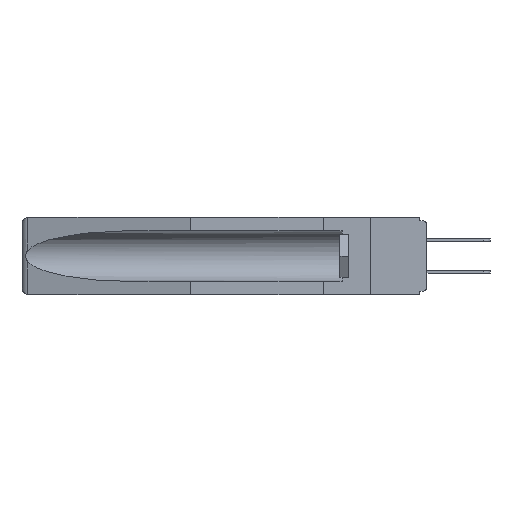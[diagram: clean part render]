
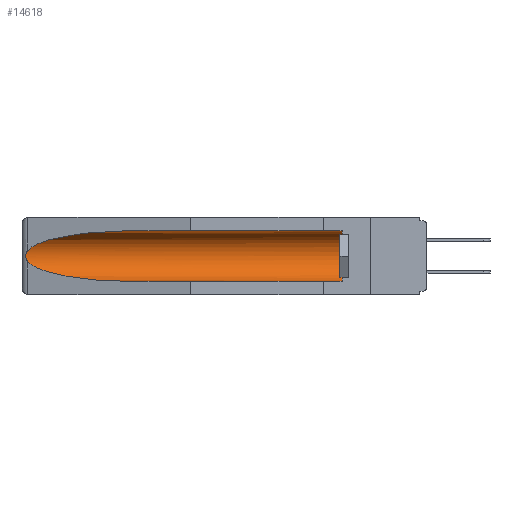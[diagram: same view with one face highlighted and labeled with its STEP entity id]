
A CAD part, left-side view. The second image highlights one B-rep face of the part: STEP entity #14618.
In plain terms, the highlighted cylindrical face has radius 2.857 mm (diameter 5.715 mm), a partial arc.
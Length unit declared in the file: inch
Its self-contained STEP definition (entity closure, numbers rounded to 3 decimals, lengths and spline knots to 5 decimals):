
#270 = CIRCLE ( 'NONE', #14272, 0.1125 ) ;
#458 = EDGE_LOOP ( 'NONE', ( #18838, #2355, #10445, #14381, #3776, #13562 ) ) ;
#537 = VECTOR ( 'NONE', #9528, 39.37008 ) ;
#879 = CARTESIAN_POINT ( 'NONE',  ( 0.26537, 1.52718, -0.14972 ) ) ;
#959 = EDGE_CURVE ( 'NONE', #11597, #9014, #8742, .T. ) ;
#1051 = VERTEX_POINT ( 'NONE', #8849 ) ;
#1425 = CARTESIAN_POINT ( 'NONE',  ( 0.21114, 1.30732, -0.059 ) ) ;
#2172 = EDGE_CURVE ( 'NONE', #1051, #14717, #2460, .T. ) ;
#2218 = CARTESIAN_POINT ( 'NONE',  ( 0.2675, 1.53308, -0.17534 ) ) ;
#2355 = ORIENTED_EDGE ( 'NONE', *, *, #12225, .T. ) ;
#2460 = LINE ( 'NONE', #17363, #537 ) ;
#2578 = DIRECTION ( 'NONE',  ( 0., 1., 0. ) ) ;
#2585 = CARTESIAN_POINT ( 'NONE',  ( 0.155, -0.30754, -0.284 ) ) ;
#3362 = VECTOR ( 'NONE', #15228, 39.37008 ) ;
#3776 = ORIENTED_EDGE ( 'NONE', *, *, #12630, .T. ) ;
#3850 = CYLINDRICAL_SURFACE ( 'NONE', #4676, 0.1125 ) ;
#4264 = CARTESIAN_POINT ( 'NONE',  ( 0.155, 0.126, -0.1715 ) ) ;
#4676 = AXIS2_PLACEMENT_3D ( 'NONE', #16590, #2578, #19429 ) ;
#5621 = CARTESIAN_POINT ( 'NONE',  ( 0.26537, 1.52718, -0.19328 ) ) ;
#6923 = CARTESIAN_POINT ( 'NONE',  ( 0.26537, 1.52718, -0.19328 ) ) ;
#7240 = CARTESIAN_POINT ( 'NONE',  ( 0.2673, 1.53269, -0.17917 ) ) ;
#7721 = CARTESIAN_POINT ( 'NONE',  ( 0.25451, 1.48313, -0.09465 ) ) ;
#8742 = LINE ( 'NONE', #2585, #3362 ) ;
#8849 = CARTESIAN_POINT ( 'NONE',  ( 0.155, 0.126, -0.059 ) ) ;
#9014 = VERTEX_POINT ( 'NONE', #11829 ) ;
#9016 = CARTESIAN_POINT ( 'NONE',  ( 0.155, 1.07973, -0.059 ) ) ;
#9295 = VERTEX_POINT ( 'NONE', #6923 ) ;
#9414 = CARTESIAN_POINT ( 'NONE',  ( 0.25451, 1.48313, -0.24835 ) ) ;
#9482 = CARTESIAN_POINT ( 'NONE',  ( 0.155, 1.07973, -0.284 ) ) ;
#9528 = DIRECTION ( 'NONE',  ( 0., 1., 0. ) ) ;
#9850 = CARTESIAN_POINT ( 'NONE',  ( 0.26597, 1.52961, -0.15275 ) ) ;
#10049 = CARTESIAN_POINT ( 'NONE',  ( 0.26654, 1.53092, -0.15636 ) ) ;
#10445 = ORIENTED_EDGE ( 'NONE', *, *, #16759, .T. ) ;
#10637 = EDGE_CURVE ( 'NONE', #14717, #15117, #18664, .T. ) ;
#11128 = CARTESIAN_POINT ( 'NONE',  ( 0.21114, 1.30732, -0.284 ) ) ;
#11597 = VERTEX_POINT ( 'NONE', #14303 ) ;
#11761 = CARTESIAN_POINT ( 'NONE',  ( 0.26597, 1.5296, -0.19026 ) ) ;
#11829 = CARTESIAN_POINT ( 'NONE',  ( 0.155, 1.07973, -0.284 ) ) ;
#12225 = EDGE_CURVE ( 'NONE', #15117, #9295, #15703, .T. ) ;
#12630 = EDGE_CURVE ( 'NONE', #11597, #1051, #270, .T. ) ;
#13419 = DIRECTION ( 'NONE',  ( 0., 0., 1. ) ) ;
#13562 = ORIENTED_EDGE ( 'NONE', *, *, #2172, .T. ) ;
#13948 = CARTESIAN_POINT ( 'NONE',  ( 0.155, 1.07973, -0.059 ) ) ;
#14272 = AXIS2_PLACEMENT_3D ( 'NONE', #4264, #16679, #13419 ) ;
#14303 = CARTESIAN_POINT ( 'NONE',  ( 0.155, 0.126, -0.284 ) ) ;
#14381 = ORIENTED_EDGE ( 'NONE', *, *, #959, .F. ) ;
#14618 = ADVANCED_FACE ( 'NONE', ( #15265 ), #3850, .F. ) ;
#14717 = VERTEX_POINT ( 'NONE', #9016 ) ;
#15085 =( BOUNDED_CURVE ( )  B_SPLINE_CURVE ( 3, ( #17177, #9414, #11128, #9482 ),
 .UNSPECIFIED., .F., .F. ) 
 B_SPLINE_CURVE_WITH_KNOTS ( ( 4, 4 ),
 ( 0.1948, 1.5708 ),
 .UNSPECIFIED. ) 
 CURVE ( )  GEOMETRIC_REPRESENTATION_ITEM ( )  RATIONAL_B_SPLINE_CURVE ( ( 1., 0.848, 0.848, 1. ) ) 
 REPRESENTATION_ITEM ( '' )  );
#15117 = VERTEX_POINT ( 'NONE', #879 ) ;
#15228 = DIRECTION ( 'NONE',  ( 0., 1., 0. ) ) ;
#15265 = FACE_OUTER_BOUND ( 'NONE', #458, .T. ) ;
#15703 = B_SPLINE_CURVE_WITH_KNOTS ( 'NONE', 3,
 ( #16106, #9850, #10049, #17662, #19211, #2218, #7240, #16642, #11761, #5621 ),
 .UNSPECIFIED., .F., .F.,
 ( 4, 2, 2, 2, 4 ),
 ( 0., 0.00029, 0.00058, 0.00087, 0.00117 ),
 .UNSPECIFIED. ) ;
#16106 = CARTESIAN_POINT ( 'NONE',  ( 0.26537, 1.52718, -0.14972 ) ) ;
#16590 = CARTESIAN_POINT ( 'NONE',  ( 0.155, -0.30754, -0.1715 ) ) ;
#16642 = CARTESIAN_POINT ( 'NONE',  ( 0.26655, 1.53094, -0.18657 ) ) ;
#16679 = DIRECTION ( 'NONE',  ( 0., -1., 0. ) ) ;
#16759 = EDGE_CURVE ( 'NONE', #9295, #9014, #15085, .T. ) ;
#17177 = CARTESIAN_POINT ( 'NONE',  ( 0.26537, 1.52718, -0.19328 ) ) ;
#17363 = CARTESIAN_POINT ( 'NONE',  ( 0.155, -0.30754, -0.059 ) ) ;
#17662 = CARTESIAN_POINT ( 'NONE',  ( 0.2673, 1.5327, -0.16383 ) ) ;
#18613 = CARTESIAN_POINT ( 'NONE',  ( 0.26537, 1.52718, -0.14972 ) ) ;
#18664 =( BOUNDED_CURVE ( )  B_SPLINE_CURVE ( 3, ( #13948, #1425, #7721, #18613 ),
 .UNSPECIFIED., .F., .T. ) 
 B_SPLINE_CURVE_WITH_KNOTS ( ( 4, 4 ),
 ( 4.71239, 6.08839 ),
 .UNSPECIFIED. ) 
 CURVE ( )  GEOMETRIC_REPRESENTATION_ITEM ( )  RATIONAL_B_SPLINE_CURVE ( ( 1., 0.848, 0.848, 1. ) ) 
 REPRESENTATION_ITEM ( '' )  );
#18838 = ORIENTED_EDGE ( 'NONE', *, *, #10637, .T. ) ;
#19211 = CARTESIAN_POINT ( 'NONE',  ( 0.2675, 1.53308, -0.16763 ) ) ;
#19429 = DIRECTION ( 'NONE',  ( 0., 0., 1. ) ) ;
